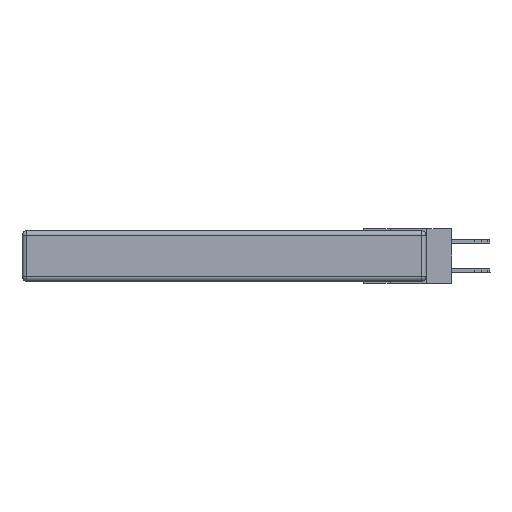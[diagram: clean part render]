
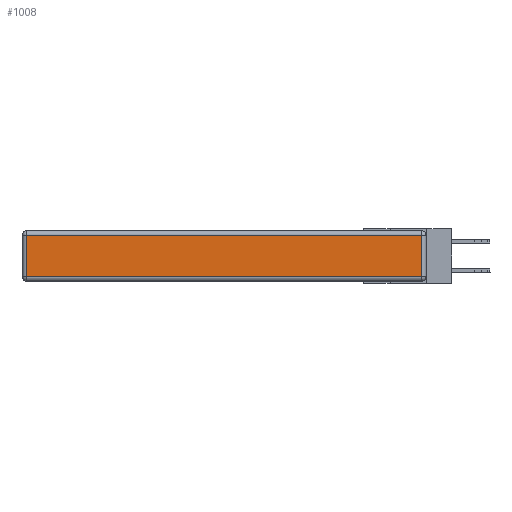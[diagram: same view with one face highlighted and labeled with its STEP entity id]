
A CAD part, left-side view. The second image highlights one B-rep face of the part: STEP entity #1008.
In plain terms, the highlighted planar face has unit normal (-1, 0, 0).
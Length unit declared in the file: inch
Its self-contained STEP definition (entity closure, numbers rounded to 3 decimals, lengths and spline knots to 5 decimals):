
#880 = DIRECTION ( 'NONE',  ( 0., 1., 0. ) ) ;
#1008 = ADVANCED_FACE ( 'NONE', ( #2357 ), #3691, .T. ) ;
#1035 = VERTEX_POINT ( 'NONE', #10329 ) ;
#1638 = LINE ( 'NONE', #3378, #10018 ) ;
#1744 = VECTOR ( 'NONE', #14534, 39.37008 ) ;
#1867 = VERTEX_POINT ( 'NONE', #4345 ) ;
#2179 = CARTESIAN_POINT ( 'NONE',  ( 0., 0.03, -0.313 ) ) ;
#2357 = FACE_OUTER_BOUND ( 'NONE', #14486, .T. ) ;
#3378 = CARTESIAN_POINT ( 'NONE',  ( 0., 2.72, -0.343 ) ) ;
#3691 = PLANE ( 'NONE',  #12223 ) ;
#4064 = VECTOR ( 'NONE', #13163, 39.37008 ) ;
#4117 = VERTEX_POINT ( 'NONE', #2179 ) ;
#4345 = CARTESIAN_POINT ( 'NONE',  ( 0., 2.72, -0.313 ) ) ;
#7103 = ORIENTED_EDGE ( 'NONE', *, *, #13510, .T. ) ;
#7353 = DIRECTION ( 'NONE',  ( -1., 0., 0. ) ) ;
#8510 = EDGE_CURVE ( 'NONE', #4117, #1035, #13115, .T. ) ;
#8631 = ORIENTED_EDGE ( 'NONE', *, *, #12817, .T. ) ;
#8751 = ORIENTED_EDGE ( 'NONE', *, *, #10184, .T. ) ;
#9277 = LINE ( 'NONE', #15690, #1744 ) ;
#10018 = VECTOR ( 'NONE', #10517, 39.37008 ) ;
#10184 = EDGE_CURVE ( 'NONE', #12786, #1867, #1638, .T. ) ;
#10329 = CARTESIAN_POINT ( 'NONE',  ( 0., 0.03, -0.03 ) ) ;
#10517 = DIRECTION ( 'NONE',  ( 0., 0., -1. ) ) ;
#11518 = CARTESIAN_POINT ( 'NONE',  ( 0., 0., -0.343 ) ) ;
#12223 = AXIS2_PLACEMENT_3D ( 'NONE', #11518, #7353, #14228 ) ;
#12786 = VERTEX_POINT ( 'NONE', #17013 ) ;
#12817 = EDGE_CURVE ( 'NONE', #1035, #12786, #17033, .T. ) ;
#13115 = LINE ( 'NONE', #15835, #4064 ) ;
#13163 = DIRECTION ( 'NONE',  ( 0., 0., 1. ) ) ;
#13510 = EDGE_CURVE ( 'NONE', #1867, #4117, #9277, .T. ) ;
#14228 = DIRECTION ( 'NONE',  ( 0., 0., 1. ) ) ;
#14486 = EDGE_LOOP ( 'NONE', ( #7103, #15229, #8631, #8751 ) ) ;
#14534 = DIRECTION ( 'NONE',  ( 0., -1., 0. ) ) ;
#14725 = VECTOR ( 'NONE', #880, 39.37008 ) ;
#15229 = ORIENTED_EDGE ( 'NONE', *, *, #8510, .T. ) ;
#15690 = CARTESIAN_POINT ( 'NONE',  ( 0., 0., -0.313 ) ) ;
#15835 = CARTESIAN_POINT ( 'NONE',  ( 0., 0.03, -0.343 ) ) ;
#17013 = CARTESIAN_POINT ( 'NONE',  ( 0., 2.72, -0.03 ) ) ;
#17033 = LINE ( 'NONE', #17076, #14725 ) ;
#17076 = CARTESIAN_POINT ( 'NONE',  ( 0., 2.75, -0.03 ) ) ;
